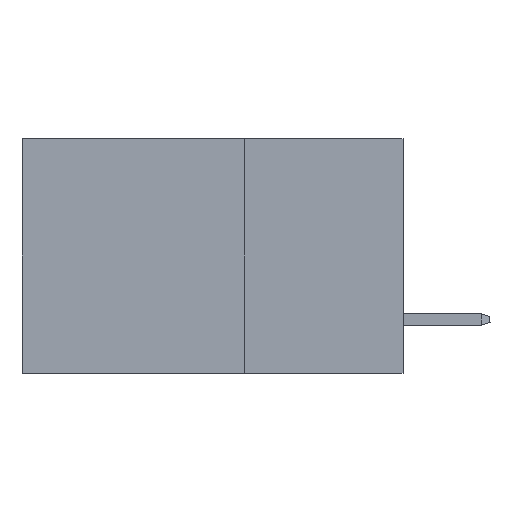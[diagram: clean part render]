
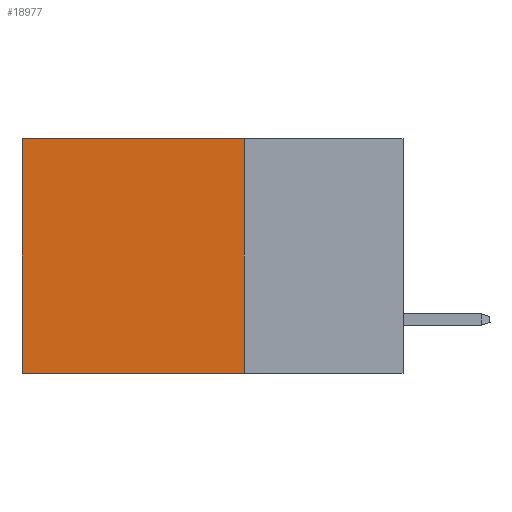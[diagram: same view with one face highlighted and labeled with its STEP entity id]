
A CAD part, left-side view. The second image highlights one B-rep face of the part: STEP entity #18977.
In plain terms, the highlighted planar face has unit normal (-1, 0, 0).
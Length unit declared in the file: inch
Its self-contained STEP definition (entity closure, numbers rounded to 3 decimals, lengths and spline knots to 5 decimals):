
#829 = LINE ( 'NONE', #7361, #18723 ) ;
#891 = ORIENTED_EDGE ( 'NONE', *, *, #11337, .F. ) ;
#932 = VECTOR ( 'NONE', #5719, 39.37008 ) ;
#1783 = ORIENTED_EDGE ( 'NONE', *, *, #20031, .T. ) ;
#2307 = DIRECTION ( 'NONE',  ( 1., 0., 0. ) ) ;
#2717 = VERTEX_POINT ( 'NONE', #6988 ) ;
#3268 = CARTESIAN_POINT ( 'NONE',  ( 0.2875, 0.6, -0.37 ) ) ;
#3648 = CARTESIAN_POINT ( 'NONE',  ( 0.2875, 0.25, 0. ) ) ;
#3712 = FACE_OUTER_BOUND ( 'NONE', #10044, .T. ) ;
#5117 = VECTOR ( 'NONE', #16416, 39.37008 ) ;
#5613 = EDGE_CURVE ( 'NONE', #10994, #2717, #19470, .T. ) ;
#5719 = DIRECTION ( 'NONE',  ( 0., 0., -1. ) ) ;
#6861 = DIRECTION ( 'NONE',  ( 0., 0., -1. ) ) ;
#6988 = CARTESIAN_POINT ( 'NONE',  ( 0.2875, 0.25, -0.37 ) ) ;
#7361 = CARTESIAN_POINT ( 'NONE',  ( 0.2875, 0.25, -0.37 ) ) ;
#7818 = AXIS2_PLACEMENT_3D ( 'NONE', #10444, #2307, #8836 ) ;
#8123 = EDGE_CURVE ( 'NONE', #9243, #19220, #15445, .T. ) ;
#8836 = DIRECTION ( 'NONE',  ( 0., 0., -1. ) ) ;
#9243 = VERTEX_POINT ( 'NONE', #20989 ) ;
#9898 = CARTESIAN_POINT ( 'NONE',  ( 0.2875, 0.25, 0. ) ) ;
#10044 = EDGE_LOOP ( 'NONE', ( #18267, #891, #20131, #1783 ) ) ;
#10444 = CARTESIAN_POINT ( 'NONE',  ( 0.2875, 0.25, 0. ) ) ;
#10994 = VERTEX_POINT ( 'NONE', #20888 ) ;
#11067 = VECTOR ( 'NONE', #6861, 39.37008 ) ;
#11337 = EDGE_CURVE ( 'NONE', #2717, #19220, #829, .T. ) ;
#12748 = DIRECTION ( 'NONE',  ( 0., 1., 0. ) ) ;
#13083 = LINE ( 'NONE', #9898, #5117 ) ;
#15242 = PLANE ( 'NONE',  #7818 ) ;
#15445 = LINE ( 'NONE', #16957, #932 ) ;
#16416 = DIRECTION ( 'NONE',  ( 0., 1., 0. ) ) ;
#16957 = CARTESIAN_POINT ( 'NONE',  ( 0.2875, 0.6, 0. ) ) ;
#18267 = ORIENTED_EDGE ( 'NONE', *, *, #8123, .T. ) ;
#18723 = VECTOR ( 'NONE', #12748, 39.37008 ) ;
#18977 = ADVANCED_FACE ( 'NONE', ( #3712 ), #15242, .F. ) ;
#19220 = VERTEX_POINT ( 'NONE', #3268 ) ;
#19470 = LINE ( 'NONE', #3648, #11067 ) ;
#20031 = EDGE_CURVE ( 'NONE', #10994, #9243, #13083, .T. ) ;
#20131 = ORIENTED_EDGE ( 'NONE', *, *, #5613, .F. ) ;
#20888 = CARTESIAN_POINT ( 'NONE',  ( 0.2875, 0.25, 0. ) ) ;
#20989 = CARTESIAN_POINT ( 'NONE',  ( 0.2875, 0.6, 0. ) ) ;
